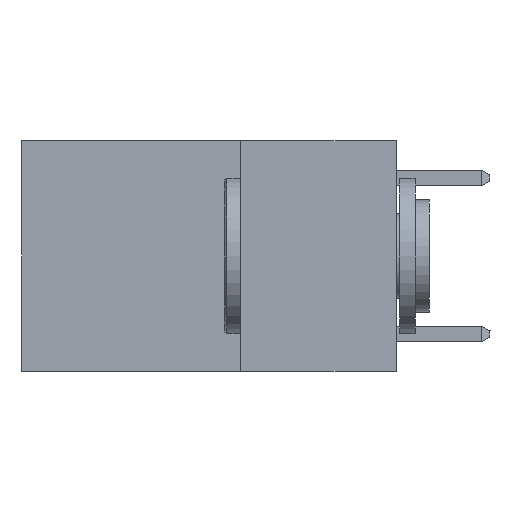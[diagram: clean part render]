
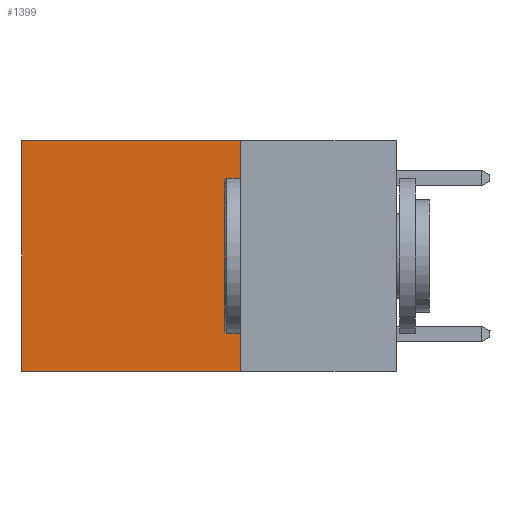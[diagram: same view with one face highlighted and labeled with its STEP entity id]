
A CAD part, left-side view. The second image highlights one B-rep face of the part: STEP entity #1399.
In plain terms, the highlighted planar face has unit normal (-1, 0, 0).
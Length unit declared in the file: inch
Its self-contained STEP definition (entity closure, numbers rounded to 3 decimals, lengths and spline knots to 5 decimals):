
#1399 = ADVANCED_FACE ( 'NONE', ( #12549 ), #1958, .F. ) ;
#1873 = ORIENTED_EDGE ( 'NONE', *, *, #5668, .T. ) ;
#1910 = CARTESIAN_POINT ( 'NONE',  ( 0.2625, 0.25, 0. ) ) ;
#1958 = PLANE ( 'NONE',  #31300 ) ;
#2696 = ORIENTED_EDGE ( 'NONE', *, *, #7460, .F. ) ;
#3276 = LINE ( 'NONE', #8825, #15875 ) ;
#3363 = CARTESIAN_POINT ( 'NONE',  ( 0.2625, 0.25, -0.37 ) ) ;
#4281 = CARTESIAN_POINT ( 'NONE',  ( 0.2625, 0.25, -0.37 ) ) ;
#5668 = EDGE_CURVE ( 'NONE', #29608, #20884, #3276, .T. ) ;
#5758 = LINE ( 'NONE', #10332, #24167 ) ;
#5912 = DIRECTION ( 'NONE',  ( 0., 1., 0. ) ) ;
#7460 = EDGE_CURVE ( 'NONE', #20767, #20884, #9897, .T. ) ;
#7742 = EDGE_LOOP ( 'NONE', ( #1873, #2696, #17635, #11786 ) ) ;
#7843 = VERTEX_POINT ( 'NONE', #29665 ) ;
#8825 = CARTESIAN_POINT ( 'NONE',  ( 0.2625, 0.6, 0. ) ) ;
#9560 = DIRECTION ( 'NONE',  ( 0., 1., 0. ) ) ;
#9897 = LINE ( 'NONE', #3363, #22396 ) ;
#10332 = CARTESIAN_POINT ( 'NONE',  ( 0.2625, 0.25, 0. ) ) ;
#11786 = ORIENTED_EDGE ( 'NONE', *, *, #30419, .T. ) ;
#12549 = FACE_OUTER_BOUND ( 'NONE', #7742, .T. ) ;
#12644 = LINE ( 'NONE', #1910, #16952 ) ;
#13719 = CARTESIAN_POINT ( 'NONE',  ( 0.2625, 0.6, 0. ) ) ;
#14629 = DIRECTION ( 'NONE',  ( 1., 0., 0. ) ) ;
#15875 = VECTOR ( 'NONE', #28756, 39.37008 ) ;
#16126 = EDGE_CURVE ( 'NONE', #7843, #20767, #5758, .T. ) ;
#16952 = VECTOR ( 'NONE', #9560, 39.37008 ) ;
#17635 = ORIENTED_EDGE ( 'NONE', *, *, #16126, .F. ) ;
#20767 = VERTEX_POINT ( 'NONE', #4281 ) ;
#20884 = VERTEX_POINT ( 'NONE', #31972 ) ;
#22396 = VECTOR ( 'NONE', #5912, 39.37008 ) ;
#24167 = VECTOR ( 'NONE', #25286, 39.37008 ) ;
#25286 = DIRECTION ( 'NONE',  ( 0., 0., -1. ) ) ;
#28756 = DIRECTION ( 'NONE',  ( 0., 0., -1. ) ) ;
#29502 = CARTESIAN_POINT ( 'NONE',  ( 0.2625, 0.25, 0. ) ) ;
#29608 = VERTEX_POINT ( 'NONE', #13719 ) ;
#29665 = CARTESIAN_POINT ( 'NONE',  ( 0.2625, 0.25, 0. ) ) ;
#30419 = EDGE_CURVE ( 'NONE', #7843, #29608, #12644, .T. ) ;
#31300 = AXIS2_PLACEMENT_3D ( 'NONE', #29502, #14629, #31878 ) ;
#31878 = DIRECTION ( 'NONE',  ( 0., 0., -1. ) ) ;
#31972 = CARTESIAN_POINT ( 'NONE',  ( 0.2625, 0.6, -0.37 ) ) ;
